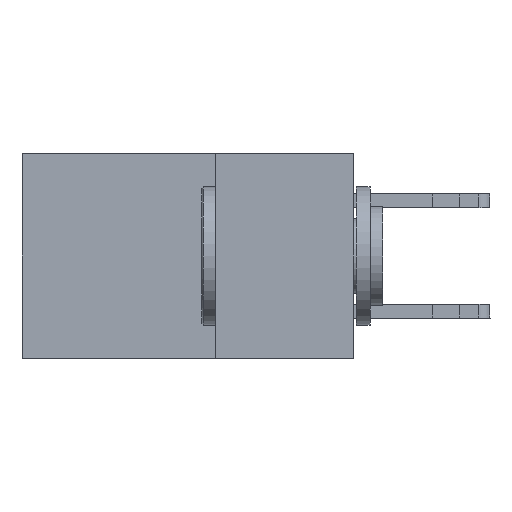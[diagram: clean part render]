
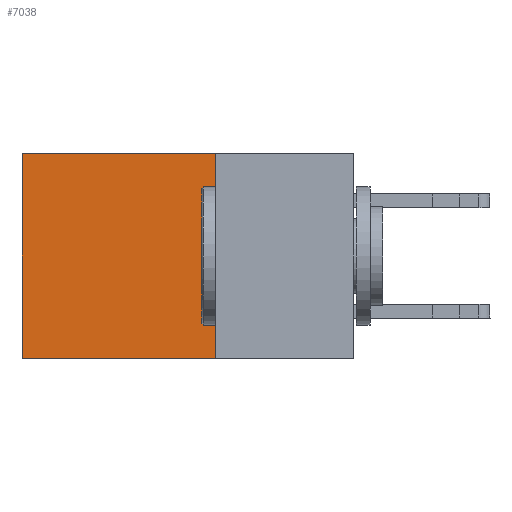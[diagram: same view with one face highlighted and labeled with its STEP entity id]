
A CAD part, left-side view. The second image highlights one B-rep face of the part: STEP entity #7038.
In plain terms, the highlighted planar face has unit normal (-1, 0, 0).
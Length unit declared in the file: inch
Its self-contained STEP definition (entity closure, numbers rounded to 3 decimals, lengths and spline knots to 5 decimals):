
#352 = ORIENTED_EDGE ( 'NONE', *, *, #28570, .F. ) ;
#899 = DIRECTION ( 'NONE',  ( 0., 1., 0. ) ) ;
#1680 = PLANE ( 'NONE',  #30973 ) ;
#2632 = DIRECTION ( 'NONE',  ( 0., 1., 0. ) ) ;
#3113 = VERTEX_POINT ( 'NONE', #12941 ) ;
#3795 = CARTESIAN_POINT ( 'NONE',  ( 0.2875, 0.25, 0. ) ) ;
#3827 = DIRECTION ( 'NONE',  ( 0., 0., -1. ) ) ;
#3997 = VERTEX_POINT ( 'NONE', #4983 ) ;
#4178 = DIRECTION ( 'NONE',  ( 1., 0., 0. ) ) ;
#4983 = CARTESIAN_POINT ( 'NONE',  ( 0.2875, 0.25, 0. ) ) ;
#6812 = EDGE_CURVE ( 'NONE', #14219, #21099, #23884, .T. ) ;
#7038 = ADVANCED_FACE ( 'NONE', ( #12867 ), #1680, .F. ) ;
#7785 = VECTOR ( 'NONE', #2632, 39.37008 ) ;
#7871 = CARTESIAN_POINT ( 'NONE',  ( 0.2875, 0.25, 0. ) ) ;
#8250 = LINE ( 'NONE', #3795, #13069 ) ;
#8531 = ORIENTED_EDGE ( 'NONE', *, *, #6812, .F. ) ;
#8548 = CARTESIAN_POINT ( 'NONE',  ( 0.2875, 0.25, -0.37 ) ) ;
#11838 = CARTESIAN_POINT ( 'NONE',  ( 0.2875, 0.6, 0. ) ) ;
#12180 = DIRECTION ( 'NONE',  ( 0., 0., -1. ) ) ;
#12867 = FACE_OUTER_BOUND ( 'NONE', #20566, .T. ) ;
#12941 = CARTESIAN_POINT ( 'NONE',  ( 0.2875, 0.6, 0. ) ) ;
#13069 = VECTOR ( 'NONE', #27352, 39.37008 ) ;
#14192 = CARTESIAN_POINT ( 'NONE',  ( 0.2875, 0.6, -0.37 ) ) ;
#14219 = VERTEX_POINT ( 'NONE', #8548 ) ;
#14675 = EDGE_CURVE ( 'NONE', #3997, #3113, #18704, .T. ) ;
#16380 = CARTESIAN_POINT ( 'NONE',  ( 0.2875, 0.25, -0.37 ) ) ;
#16918 = VECTOR ( 'NONE', #899, 39.37008 ) ;
#17051 = CARTESIAN_POINT ( 'NONE',  ( 0.2875, 0.25, 0. ) ) ;
#18704 = LINE ( 'NONE', #7871, #7785 ) ;
#19220 = EDGE_CURVE ( 'NONE', #3113, #21099, #21191, .T. ) ;
#20174 = ORIENTED_EDGE ( 'NONE', *, *, #14675, .T. ) ;
#20566 = EDGE_LOOP ( 'NONE', ( #24718, #8531, #352, #20174 ) ) ;
#21099 = VERTEX_POINT ( 'NONE', #14192 ) ;
#21191 = LINE ( 'NONE', #11838, #27714 ) ;
#23884 = LINE ( 'NONE', #16380, #16918 ) ;
#24718 = ORIENTED_EDGE ( 'NONE', *, *, #19220, .T. ) ;
#27352 = DIRECTION ( 'NONE',  ( 0., 0., -1. ) ) ;
#27714 = VECTOR ( 'NONE', #3827, 39.37008 ) ;
#28570 = EDGE_CURVE ( 'NONE', #3997, #14219, #8250, .T. ) ;
#30973 = AXIS2_PLACEMENT_3D ( 'NONE', #17051, #4178, #12180 ) ;
